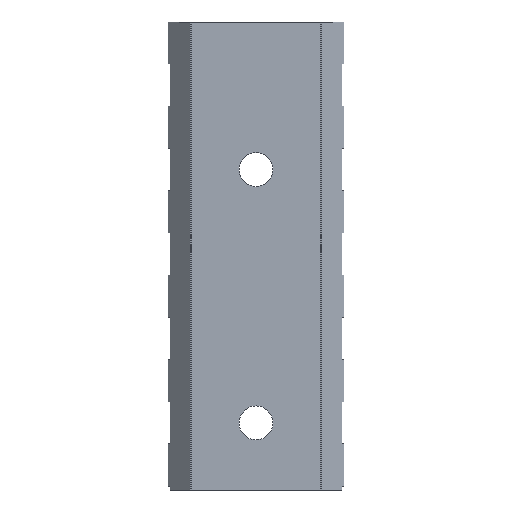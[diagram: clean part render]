
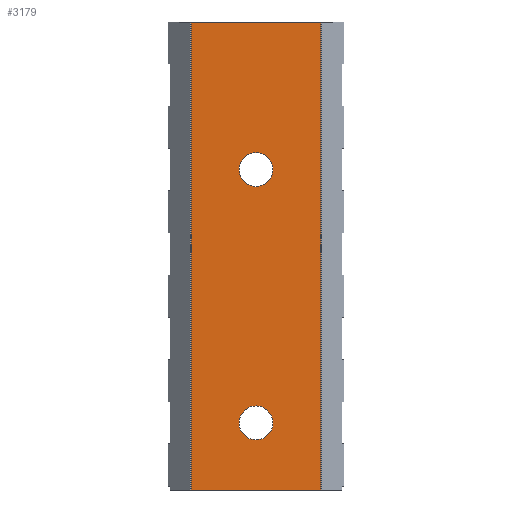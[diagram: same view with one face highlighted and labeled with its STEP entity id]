
A CAD part, front view. The second image highlights one B-rep face of the part: STEP entity #3179.
In plain terms, the highlighted planar face has unit normal (0, -1, 0).
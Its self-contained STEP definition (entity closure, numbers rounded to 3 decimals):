
#43 = PLANE('',#44);
#44 = AXIS2_PLACEMENT_3D('',#45,#46,#47);
#45 = CARTESIAN_POINT('',(16.498,9.322,-62.826));
#46 = DIRECTION('',(0.,0.,-1.));
#47 = DIRECTION('',(-1.,0.,0.));
#70 = PLANE('',#71);
#71 = AXIS2_PLACEMENT_3D('',#72,#73,#74);
#72 = CARTESIAN_POINT('',(8.,4.064,-31.368));
#73 = DIRECTION('',(-1.,0.,0.));
#74 = DIRECTION('',(0.,-1.,0.));
#96 = PLANE('',#97);
#97 = AXIS2_PLACEMENT_3D('',#98,#99,#100);
#98 = CARTESIAN_POINT('',(-15.729,9.322,-120.817));
#99 = DIRECTION('',(0.,0.,1.));
#100 = DIRECTION('',(1.,0.,0.));
#290 = VERTEX_POINT('',#291);
#291 = CARTESIAN_POINT('',(8.,-2.161,-62.826));
#310 = EDGE_CURVE('',#290,#311,#313,.T.);
#311 = VERTEX_POINT('',#312);
#312 = CARTESIAN_POINT('',(-8.,-2.161,-62.826));
#313 = SURFACE_CURVE('',#314,(#318,#324),.PCURVE_S1.);
#314 = LINE('',#315,#316);
#315 = CARTESIAN_POINT('',(12.249,-2.161,-62.826));
#316 = VECTOR('',#317,1.);
#317 = DIRECTION('',(-1.,0.,0.));
#318 = PCURVE('',#43,#319);
#319 = DEFINITIONAL_REPRESENTATION('',(#320),#323);
#320 = B_SPLINE_CURVE_WITH_KNOTS('',1,(#321,#322),.UNSPECIFIED.,.F.,.F.,
  (2,2),(2.649,21.849),.PIECEWISE_BEZIER_KNOTS.);
#321 = CARTESIAN_POINT('',(6.898,-11.483));
#322 = CARTESIAN_POINT('',(26.098,-11.483));
#323 = ( GEOMETRIC_REPRESENTATION_CONTEXT(2) 
PARAMETRIC_REPRESENTATION_CONTEXT() REPRESENTATION_CONTEXT('2D SPACE',''
  ) );
#324 = PCURVE('',#325,#330);
#325 = PLANE('',#326);
#326 = AXIS2_PLACEMENT_3D('',#327,#328,#329);
#327 = CARTESIAN_POINT('',(8.,-2.161,-31.368));
#328 = DIRECTION('',(0.,1.,0.));
#329 = DIRECTION('',(-1.,0.,0.));
#330 = DEFINITIONAL_REPRESENTATION('',(#331),#334);
#331 = B_SPLINE_CURVE_WITH_KNOTS('',1,(#332,#333),.UNSPECIFIED.,.F.,.F.,
  (2,2),(2.649,21.849),.PIECEWISE_BEZIER_KNOTS.);
#332 = CARTESIAN_POINT('',(-1.6,-31.458));
#333 = CARTESIAN_POINT('',(17.6,-31.458));
#334 = ( GEOMETRIC_REPRESENTATION_CONTEXT(2) 
PARAMETRIC_REPRESENTATION_CONTEXT() REPRESENTATION_CONTEXT('2D SPACE',''
  ) );
#351 = PLANE('',#352);
#352 = AXIS2_PLACEMENT_3D('',#353,#354,#355);
#353 = CARTESIAN_POINT('',(-8.,-2.161,-31.368));
#354 = DIRECTION('',(1.,0.,0.));
#355 = DIRECTION('',(0.,1.,0.));
#916 = VERTEX_POINT('',#917);
#917 = CARTESIAN_POINT('',(-8.,-2.161,-120.817));
#936 = EDGE_CURVE('',#916,#937,#939,.T.);
#937 = VERTEX_POINT('',#938);
#938 = CARTESIAN_POINT('',(8.,-2.161,-120.817));
#939 = SURFACE_CURVE('',#940,(#944,#950),.PCURVE_S1.);
#940 = LINE('',#941,#942);
#941 = CARTESIAN_POINT('',(-3.865,-2.161,-120.817));
#942 = VECTOR('',#943,1.);
#943 = DIRECTION('',(1.,0.,0.));
#944 = PCURVE('',#96,#945);
#945 = DEFINITIONAL_REPRESENTATION('',(#946),#949);
#946 = B_SPLINE_CURVE_WITH_KNOTS('',1,(#947,#948),.UNSPECIFIED.,.F.,.F.,
  (2,2),(-5.735,13.465),.PIECEWISE_BEZIER_KNOTS.);
#947 = CARTESIAN_POINT('',(6.129,-11.483));
#948 = CARTESIAN_POINT('',(25.329,-11.483));
#949 = ( GEOMETRIC_REPRESENTATION_CONTEXT(2) 
PARAMETRIC_REPRESENTATION_CONTEXT() REPRESENTATION_CONTEXT('2D SPACE',''
  ) );
#950 = PCURVE('',#325,#951);
#951 = DEFINITIONAL_REPRESENTATION('',(#952),#955);
#952 = B_SPLINE_CURVE_WITH_KNOTS('',1,(#953,#954),.UNSPECIFIED.,.F.,.F.,
  (2,2),(-5.735,13.465),.PIECEWISE_BEZIER_KNOTS.);
#953 = CARTESIAN_POINT('',(17.6,-89.449));
#954 = CARTESIAN_POINT('',(-1.6,-89.449));
#955 = ( GEOMETRIC_REPRESENTATION_CONTEXT(2) 
PARAMETRIC_REPRESENTATION_CONTEXT() REPRESENTATION_CONTEXT('2D SPACE',''
  ) );
#979 = EDGE_CURVE('',#290,#937,#980,.T.);
#980 = SURFACE_CURVE('',#981,(#985,#992),.PCURVE_S1.);
#981 = LINE('',#982,#983);
#982 = CARTESIAN_POINT('',(8.,-2.161,-31.368));
#983 = VECTOR('',#984,1.);
#984 = DIRECTION('',(0.,0.,-1.));
#985 = PCURVE('',#70,#986);
#986 = DEFINITIONAL_REPRESENTATION('',(#987),#991);
#987 = LINE('',#988,#989);
#988 = CARTESIAN_POINT('',(6.225,0.));
#989 = VECTOR('',#990,1.);
#990 = DIRECTION('',(0.,-1.));
#991 = ( GEOMETRIC_REPRESENTATION_CONTEXT(2) 
PARAMETRIC_REPRESENTATION_CONTEXT() REPRESENTATION_CONTEXT('2D SPACE',''
  ) );
#992 = PCURVE('',#325,#993);
#993 = DEFINITIONAL_REPRESENTATION('',(#994),#998);
#994 = LINE('',#995,#996);
#995 = CARTESIAN_POINT('',(0.,0.));
#996 = VECTOR('',#997,1.);
#997 = DIRECTION('',(0.,-1.));
#998 = ( GEOMETRIC_REPRESENTATION_CONTEXT(2) 
PARAMETRIC_REPRESENTATION_CONTEXT() REPRESENTATION_CONTEXT('2D SPACE',''
  ) );
#3157 = EDGE_CURVE('',#311,#916,#3158,.T.);
#3158 = SURFACE_CURVE('',#3159,(#3163,#3170),.PCURVE_S1.);
#3159 = LINE('',#3160,#3161);
#3160 = CARTESIAN_POINT('',(-8.,-2.161,-31.368));
#3161 = VECTOR('',#3162,1.);
#3162 = DIRECTION('',(0.,0.,-1.));
#3163 = PCURVE('',#351,#3164);
#3164 = DEFINITIONAL_REPRESENTATION('',(#3165),#3169);
#3165 = LINE('',#3166,#3167);
#3166 = CARTESIAN_POINT('',(0.,0.));
#3167 = VECTOR('',#3168,1.);
#3168 = DIRECTION('',(0.,-1.));
#3169 = ( GEOMETRIC_REPRESENTATION_CONTEXT(2) 
PARAMETRIC_REPRESENTATION_CONTEXT() REPRESENTATION_CONTEXT('2D SPACE',''
  ) );
#3170 = PCURVE('',#325,#3171);
#3171 = DEFINITIONAL_REPRESENTATION('',(#3172),#3176);
#3172 = LINE('',#3173,#3174);
#3173 = CARTESIAN_POINT('',(16.,0.));
#3174 = VECTOR('',#3175,1.);
#3175 = DIRECTION('',(0.,-1.));
#3176 = ( GEOMETRIC_REPRESENTATION_CONTEXT(2) 
PARAMETRIC_REPRESENTATION_CONTEXT() REPRESENTATION_CONTEXT('2D SPACE',''
  ) );
#3179 = ADVANCED_FACE('',(#3180,#3186,#3217),#325,.F.);
#3180 = FACE_BOUND('',#3181,.F.);
#3181 = EDGE_LOOP('',(#3182,#3183,#3184,#3185));
#3182 = ORIENTED_EDGE('',*,*,#310,.F.);
#3183 = ORIENTED_EDGE('',*,*,#979,.T.);
#3184 = ORIENTED_EDGE('',*,*,#936,.F.);
#3185 = ORIENTED_EDGE('',*,*,#3157,.F.);
#3186 = FACE_BOUND('',#3187,.F.);
#3187 = EDGE_LOOP('',(#3188));
#3188 = ORIENTED_EDGE('',*,*,#3189,.F.);
#3189 = EDGE_CURVE('',#3190,#3190,#3192,.T.);
#3190 = VERTEX_POINT('',#3191);
#3191 = CARTESIAN_POINT('',(-2.1,-2.161,-112.504));
#3192 = SURFACE_CURVE('',#3193,(#3198,#3205),.PCURVE_S1.);
#3193 = CIRCLE('',#3194,2.1);
#3194 = AXIS2_PLACEMENT_3D('',#3195,#3196,#3197);
#3195 = CARTESIAN_POINT('',(0.,-2.161,-112.504));
#3196 = DIRECTION('',(0.,1.,0.));
#3197 = DIRECTION('',(-1.,0.,0.));
#3198 = PCURVE('',#325,#3199);
#3199 = DEFINITIONAL_REPRESENTATION('',(#3200),#3204);
#3200 = CIRCLE('',#3201,2.1);
#3201 = AXIS2_PLACEMENT_2D('',#3202,#3203);
#3202 = CARTESIAN_POINT('',(8.,-81.135));
#3203 = DIRECTION('',(1.,0.));
#3204 = ( GEOMETRIC_REPRESENTATION_CONTEXT(2) 
PARAMETRIC_REPRESENTATION_CONTEXT() REPRESENTATION_CONTEXT('2D SPACE',''
  ) );
#3205 = PCURVE('',#3206,#3211);
#3206 = CYLINDRICAL_SURFACE('',#3207,2.1);
#3207 = AXIS2_PLACEMENT_3D('',#3208,#3209,#3210);
#3208 = CARTESIAN_POINT('',(0.,2.325,-112.504));
#3209 = DIRECTION('',(0.,1.,0.));
#3210 = DIRECTION('',(-1.,0.,0.));
#3211 = DEFINITIONAL_REPRESENTATION('',(#3212),#3216);
#3212 = LINE('',#3213,#3214);
#3213 = CARTESIAN_POINT('',(0.,-4.486));
#3214 = VECTOR('',#3215,1.);
#3215 = DIRECTION('',(1.,0.));
#3216 = ( GEOMETRIC_REPRESENTATION_CONTEXT(2) 
PARAMETRIC_REPRESENTATION_CONTEXT() REPRESENTATION_CONTEXT('2D SPACE',''
  ) );
#3217 = FACE_BOUND('',#3218,.F.);
#3218 = EDGE_LOOP('',(#3219));
#3219 = ORIENTED_EDGE('',*,*,#3220,.F.);
#3220 = EDGE_CURVE('',#3221,#3221,#3223,.T.);
#3221 = VERTEX_POINT('',#3222);
#3222 = CARTESIAN_POINT('',(-2.1,-2.161,-81.121));
#3223 = SURFACE_CURVE('',#3224,(#3229,#3236),.PCURVE_S1.);
#3224 = CIRCLE('',#3225,2.1);
#3225 = AXIS2_PLACEMENT_3D('',#3226,#3227,#3228);
#3226 = CARTESIAN_POINT('',(0.,-2.161,-81.121));
#3227 = DIRECTION('',(0.,1.,0.));
#3228 = DIRECTION('',(-1.,0.,0.));
#3229 = PCURVE('',#325,#3230);
#3230 = DEFINITIONAL_REPRESENTATION('',(#3231),#3235);
#3231 = CIRCLE('',#3232,2.1);
#3232 = AXIS2_PLACEMENT_2D('',#3233,#3234);
#3233 = CARTESIAN_POINT('',(8.,-49.752));
#3234 = DIRECTION('',(1.,0.));
#3235 = ( GEOMETRIC_REPRESENTATION_CONTEXT(2) 
PARAMETRIC_REPRESENTATION_CONTEXT() REPRESENTATION_CONTEXT('2D SPACE',''
  ) );
#3236 = PCURVE('',#3237,#3242);
#3237 = CYLINDRICAL_SURFACE('',#3238,2.1);
#3238 = AXIS2_PLACEMENT_3D('',#3239,#3240,#3241);
#3239 = CARTESIAN_POINT('',(0.,2.325,-81.121));
#3240 = DIRECTION('',(0.,1.,0.));
#3241 = DIRECTION('',(-1.,0.,0.));
#3242 = DEFINITIONAL_REPRESENTATION('',(#3243),#3247);
#3243 = LINE('',#3244,#3245);
#3244 = CARTESIAN_POINT('',(0.,-4.486));
#3245 = VECTOR('',#3246,1.);
#3246 = DIRECTION('',(1.,0.));
#3247 = ( GEOMETRIC_REPRESENTATION_CONTEXT(2) 
PARAMETRIC_REPRESENTATION_CONTEXT() REPRESENTATION_CONTEXT('2D SPACE',''
  ) );
